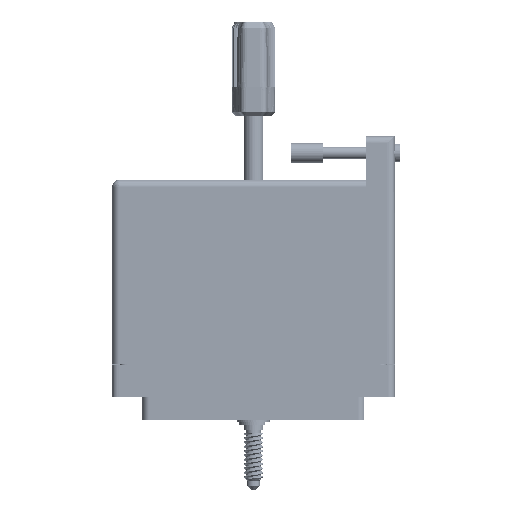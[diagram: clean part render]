
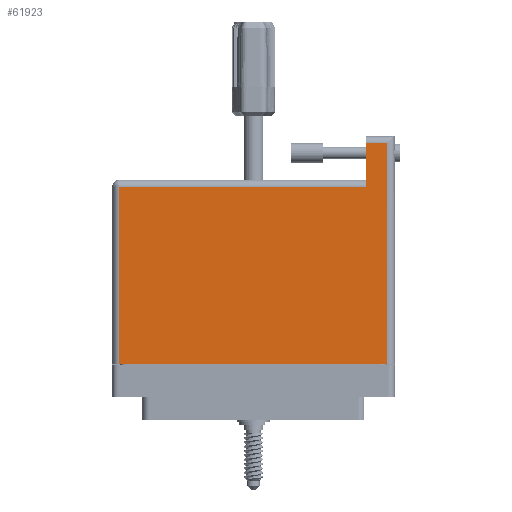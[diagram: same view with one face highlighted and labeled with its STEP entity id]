
A CAD part, front view. The second image highlights one B-rep face of the part: STEP entity #61923.
In plain terms, the highlighted face is planar.
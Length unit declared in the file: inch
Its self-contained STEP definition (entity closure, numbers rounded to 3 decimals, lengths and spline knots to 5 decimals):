
#615 = CARTESIAN_POINT ( 'NONE',  ( -1.289, -0.1, 0.617 ) ) ;
#1603 = CARTESIAN_POINT ( 'NONE',  ( -1.289, -0.1, 0.617 ) ) ;
#2543 = CARTESIAN_POINT ( 'NONE',  ( -1.359, -0.1, 0.617 ) ) ;
#2770 = PLANE ( 'NONE',  #30876 ) ;
#4101 = CARTESIAN_POINT ( 'NONE',  ( 1.289, 2.095, 0.617 ) ) ;
#4400 = DIRECTION ( 'NONE',  ( -1., 0., 0. ) ) ;
#5575 = EDGE_LOOP ( 'NONE', ( #10818, #23725, #75826, #48255, #6099, #18467 ) ) ;
#5634 = VERTEX_POINT ( 'NONE', #1603 ) ;
#6099 = ORIENTED_EDGE ( 'NONE', *, *, #63824, .T. ) ;
#6568 = CARTESIAN_POINT ( 'NONE',  ( 1.289, -0.1, 0.617 ) ) ;
#10818 = ORIENTED_EDGE ( 'NONE', *, *, #74581, .T. ) ;
#15296 = DIRECTION ( 'NONE',  ( 1., 0., 0. ) ) ;
#17570 = LINE ( 'NONE', #84621, #39311 ) ;
#18467 = ORIENTED_EDGE ( 'NONE', *, *, #19380, .T. ) ;
#19380 = EDGE_CURVE ( 'NONE', #34873, #65133, #35694, .T. ) ;
#20368 = LINE ( 'NONE', #615, #82036 ) ;
#20793 = DIRECTION ( 'NONE',  ( 0., -1., 0. ) ) ;
#22073 = EDGE_CURVE ( 'NONE', #62575, #27589, #44444, .T. ) ;
#22390 = CARTESIAN_POINT ( 'NONE',  ( -1.289, 1.605, 0.617 ) ) ;
#23725 = ORIENTED_EDGE ( 'NONE', *, *, #73532, .T. ) ;
#24370 = VECTOR ( 'NONE', #43113, 39.37008 ) ;
#27589 = VERTEX_POINT ( 'NONE', #75092 ) ;
#29552 = CARTESIAN_POINT ( 'NONE',  ( 1.079, 2.095, 0.617 ) ) ;
#30383 = CARTESIAN_POINT ( 'NONE',  ( -1.359, 1.675, 0.617 ) ) ;
#30864 = DIRECTION ( 'NONE',  ( 0., 1., 0. ) ) ;
#30876 = AXIS2_PLACEMENT_3D ( 'NONE', #30383, #57120, #77712 ) ;
#34873 = VERTEX_POINT ( 'NONE', #60985 ) ;
#34928 = CARTESIAN_POINT ( 'NONE',  ( -1.359, 1.605, 0.617 ) ) ;
#35355 = LINE ( 'NONE', #34928, #41610 ) ;
#35694 = LINE ( 'NONE', #29552, #24370 ) ;
#36907 = EDGE_CURVE ( 'NONE', #5634, #62575, #63484, .T. ) ;
#39311 = VECTOR ( 'NONE', #4400, 39.37008 ) ;
#41610 = VECTOR ( 'NONE', #62097, 39.37008 ) ;
#42639 = VERTEX_POINT ( 'NONE', #22390 ) ;
#43113 = DIRECTION ( 'NONE',  ( 0., -1., 0. ) ) ;
#44444 = LINE ( 'NONE', #4101, #44475 ) ;
#44475 = VECTOR ( 'NONE', #30864, 39.37008 ) ;
#48255 = ORIENTED_EDGE ( 'NONE', *, *, #22073, .T. ) ;
#51512 = VECTOR ( 'NONE', #15296, 39.37008 ) ;
#57120 = DIRECTION ( 'NONE',  ( 0., 0., -1. ) ) ;
#60985 = CARTESIAN_POINT ( 'NONE',  ( 1.079, 2.025, 0.617 ) ) ;
#61923 = ADVANCED_FACE ( 'NONE', ( #76416 ), #2770, .F. ) ;
#62097 = DIRECTION ( 'NONE',  ( -1., 0., 0. ) ) ;
#62575 = VERTEX_POINT ( 'NONE', #6568 ) ;
#63484 = LINE ( 'NONE', #2543, #51512 ) ;
#63824 = EDGE_CURVE ( 'NONE', #27589, #34873, #17570, .T. ) ;
#65133 = VERTEX_POINT ( 'NONE', #69761 ) ;
#69761 = CARTESIAN_POINT ( 'NONE',  ( 1.079, 1.605, 0.617 ) ) ;
#73532 = EDGE_CURVE ( 'NONE', #42639, #5634, #20368, .T. ) ;
#74581 = EDGE_CURVE ( 'NONE', #65133, #42639, #35355, .T. ) ;
#75092 = CARTESIAN_POINT ( 'NONE',  ( 1.289, 2.025, 0.617 ) ) ;
#75826 = ORIENTED_EDGE ( 'NONE', *, *, #36907, .T. ) ;
#76416 = FACE_OUTER_BOUND ( 'NONE', #5575, .T. ) ;
#77712 = DIRECTION ( 'NONE',  ( -1., 0., 0. ) ) ;
#82036 = VECTOR ( 'NONE', #20793, 39.37008 ) ;
#84621 = CARTESIAN_POINT ( 'NONE',  ( -1.359, 2.025, 0.617 ) ) ;
